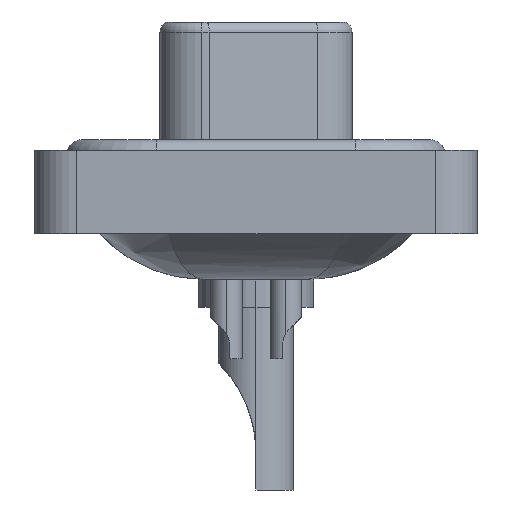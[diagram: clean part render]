
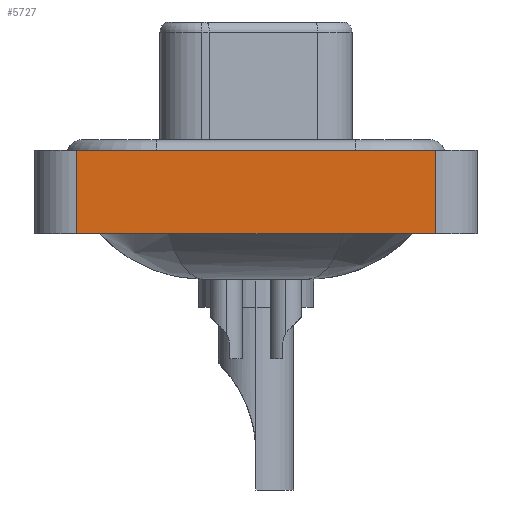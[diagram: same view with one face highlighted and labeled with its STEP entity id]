
A CAD part, left-side view. The second image highlights one B-rep face of the part: STEP entity #5727.
In plain terms, the highlighted planar face has unit normal (-1, 0, 0).
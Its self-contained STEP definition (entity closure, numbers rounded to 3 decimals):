
#260 = EDGE_CURVE ( 'NONE', #901, #4329, #9273, .T. ) ;
#766 = ORIENTED_EDGE ( 'NONE', *, *, #15907, .F. ) ;
#901 = VERTEX_POINT ( 'NONE', #20895 ) ;
#1013 = VERTEX_POINT ( 'NONE', #19585 ) ;
#1085 = DIRECTION ( 'NONE',  ( 0., 0., 1. ) ) ;
#2878 = CARTESIAN_POINT ( 'NONE',  ( -7.3, -8.55, -3.6 ) ) ;
#3103 = LINE ( 'NONE', #6028, #17900 ) ;
#4329 = VERTEX_POINT ( 'NONE', #17494 ) ;
#5727 = ADVANCED_FACE ( 'NONE', ( #8304 ), #18221, .T. ) ;
#6028 = CARTESIAN_POINT ( 'NONE',  ( -7.3, 8.55, -3.6 ) ) ;
#6357 = ORIENTED_EDGE ( 'NONE', *, *, #260, .T. ) ;
#6684 = ORIENTED_EDGE ( 'NONE', *, *, #16326, .T. ) ;
#7457 = AXIS2_PLACEMENT_3D ( 'NONE', #11336, #14586, #12947 ) ;
#7881 = CARTESIAN_POINT ( 'NONE',  ( -7.3, 8.55, 0.4 ) ) ;
#8304 = FACE_OUTER_BOUND ( 'NONE', #20255, .T. ) ;
#8840 = CARTESIAN_POINT ( 'NONE',  ( -7.3, -8.55, -3.6 ) ) ;
#9273 = LINE ( 'NONE', #8840, #12389 ) ;
#11179 = DIRECTION ( 'NONE',  ( 0., 0., 1. ) ) ;
#11267 = EDGE_CURVE ( 'NONE', #901, #20718, #3103, .T. ) ;
#11336 = CARTESIAN_POINT ( 'NONE',  ( -7.3, -8.55, -3.6 ) ) ;
#12184 = DIRECTION ( 'NONE',  ( 0., -1., 0. ) ) ;
#12389 = VECTOR ( 'NONE', #12184, 1000. ) ;
#12537 = CARTESIAN_POINT ( 'NONE',  ( -7.3, -8.55, 0.4 ) ) ;
#12947 = DIRECTION ( 'NONE',  ( 0., 0., 1. ) ) ;
#14586 = DIRECTION ( 'NONE',  ( -1., 0., 0. ) ) ;
#14849 = LINE ( 'NONE', #2878, #16632 ) ;
#15907 = EDGE_CURVE ( 'NONE', #20718, #1013, #20724, .T. ) ;
#16326 = EDGE_CURVE ( 'NONE', #4329, #1013, #14849, .T. ) ;
#16632 = VECTOR ( 'NONE', #11179, 1000. ) ;
#17494 = CARTESIAN_POINT ( 'NONE',  ( -7.3, -8.55, -3.6 ) ) ;
#17517 = ORIENTED_EDGE ( 'NONE', *, *, #11267, .F. ) ;
#17900 = VECTOR ( 'NONE', #1085, 1000. ) ;
#18221 = PLANE ( 'NONE',  #7457 ) ;
#18344 = VECTOR ( 'NONE', #19212, 1000. ) ;
#19212 = DIRECTION ( 'NONE',  ( 0., -1., 0. ) ) ;
#19585 = CARTESIAN_POINT ( 'NONE',  ( -7.3, -8.55, 0.4 ) ) ;
#20255 = EDGE_LOOP ( 'NONE', ( #6684, #766, #17517, #6357 ) ) ;
#20718 = VERTEX_POINT ( 'NONE', #7881 ) ;
#20724 = LINE ( 'NONE', #12537, #18344 ) ;
#20895 = CARTESIAN_POINT ( 'NONE',  ( -7.3, 8.55, -3.6 ) ) ;
